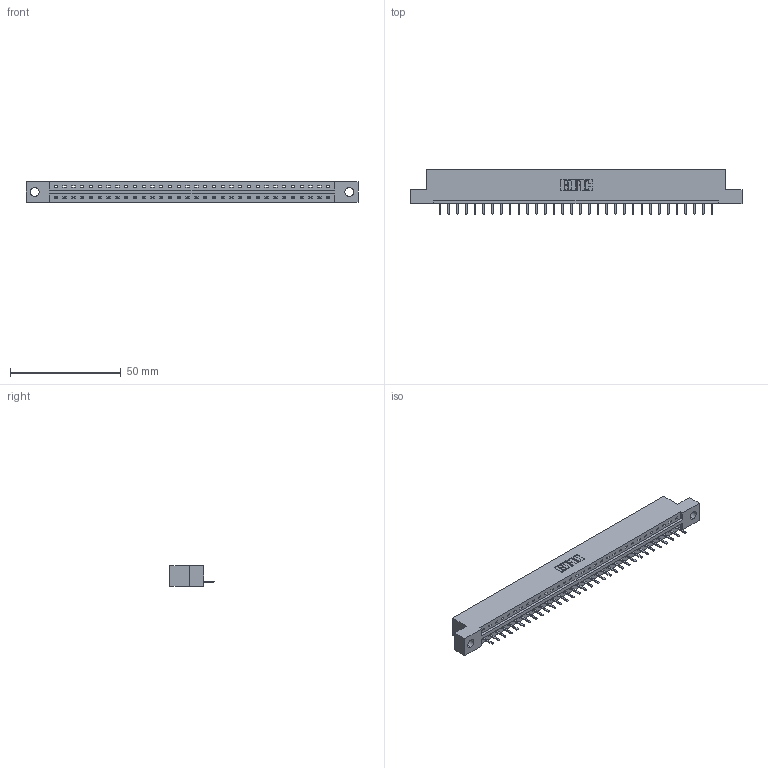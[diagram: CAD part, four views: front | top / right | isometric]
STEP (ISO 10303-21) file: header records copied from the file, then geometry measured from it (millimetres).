
FILE_DESCRIPTION (( 'STEP AP203' ), '1' );
FILE_NAME ('387-032-520-104.STEP', '2018-09-18T05:25:03', ( '' ), ( '' ), 'SwSTEP 2.0', 'SolidWorks 2016', '' );
FILE_SCHEMA (( 'CONFIG_CONTROL_DESIGN' ));
Length unit declared in the file: inch
Products named in the file (3): 345-292-001_345-293-120; 387-032-520-104; 337 Part_Flush Mounting Lugs - 0.156 Dia-TH
Assembly tree (33 placements, depth 2):
  387-032-520-104
    337 Part_Flush Mounting Lugs - 0.156 Dia-TH
    345-292-001_345-293-120  x32
Bounding box: 149.81 x 20.02 x 9.4 mm (x, y, z)
Volume: 15265.1 mm3; surface area: 15182.7 mm2
Topology: 33 solids, 33 shells, 2226 faces, 6583 edges, 4302 vertices
Faces by surface type: plane 1606, cylinder 620
Entity records: 25197 total; most frequent: CARTESIAN_POINT 4406, ORIENTED_EDGE 4362, DIRECTION 3717, EDGE_CURVE 2181, LINE 2049, VECTOR 2049, VERTEX_POINT 1450, AXIS2_PLACEMENT_3D 834
